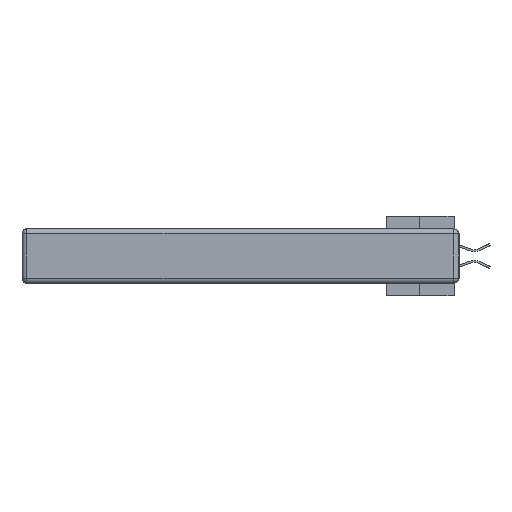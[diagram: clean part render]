
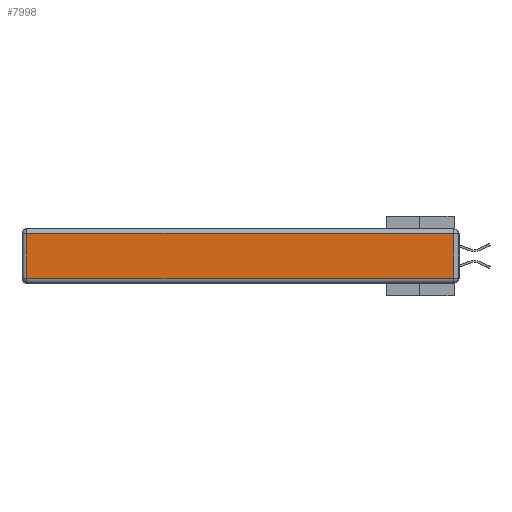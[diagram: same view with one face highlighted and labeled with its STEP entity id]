
A CAD part, left-side view. The second image highlights one B-rep face of the part: STEP entity #7998.
In plain terms, the highlighted planar face has unit normal (-1, 0, 0).
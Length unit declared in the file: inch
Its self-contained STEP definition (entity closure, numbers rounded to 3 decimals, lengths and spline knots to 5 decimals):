
#637 = VERTEX_POINT ( 'NONE', #21173 ) ;
#3758 = LINE ( 'NONE', #36988, #16780 ) ;
#6068 = CARTESIAN_POINT ( 'NONE',  ( 0., 0., -0.313 ) ) ;
#6071 = VECTOR ( 'NONE', #31229, 39.37008 ) ;
#6624 = VERTEX_POINT ( 'NONE', #7556 ) ;
#7320 = LINE ( 'NONE', #24693, #14681 ) ;
#7408 = ORIENTED_EDGE ( 'NONE', *, *, #41758, .T. ) ;
#7542 = CARTESIAN_POINT ( 'NONE',  ( 0., 0., -0.343 ) ) ;
#7556 = CARTESIAN_POINT ( 'NONE',  ( 0., 0.03, -0.03 ) ) ;
#7998 = ADVANCED_FACE ( 'NONE', ( #30467 ), #21424, .T. ) ;
#9216 = LINE ( 'NONE', #45292, #31706 ) ;
#9515 = DIRECTION ( 'NONE',  ( 0., 1., 0. ) ) ;
#10501 = DIRECTION ( 'NONE',  ( -1., 0., 0. ) ) ;
#10829 = DIRECTION ( 'NONE',  ( 0., 0., 1. ) ) ;
#14134 = EDGE_CURVE ( 'NONE', #637, #38287, #3758, .T. ) ;
#14681 = VECTOR ( 'NONE', #41924, 39.37008 ) ;
#16780 = VECTOR ( 'NONE', #43570, 39.37008 ) ;
#19250 = AXIS2_PLACEMENT_3D ( 'NONE', #7542, #10501, #10829 ) ;
#20720 = EDGE_CURVE ( 'NONE', #38287, #21217, #45965, .T. ) ;
#21173 = CARTESIAN_POINT ( 'NONE',  ( 0., 2.72, -0.03 ) ) ;
#21217 = VERTEX_POINT ( 'NONE', #27257 ) ;
#21424 = PLANE ( 'NONE',  #19250 ) ;
#24693 = CARTESIAN_POINT ( 'NONE',  ( 0., 0.03, -0.343 ) ) ;
#25277 = ORIENTED_EDGE ( 'NONE', *, *, #20720, .T. ) ;
#27257 = CARTESIAN_POINT ( 'NONE',  ( 0., 0.03, -0.313 ) ) ;
#28743 = CARTESIAN_POINT ( 'NONE',  ( 0., 2.72, -0.313 ) ) ;
#30467 = FACE_OUTER_BOUND ( 'NONE', #36541, .T. ) ;
#31229 = DIRECTION ( 'NONE',  ( 0., -1., 0. ) ) ;
#31706 = VECTOR ( 'NONE', #9515, 39.37008 ) ;
#36541 = EDGE_LOOP ( 'NONE', ( #25277, #42987, #7408, #43739 ) ) ;
#36988 = CARTESIAN_POINT ( 'NONE',  ( 0., 2.72, -0.343 ) ) ;
#37415 = EDGE_CURVE ( 'NONE', #21217, #6624, #7320, .T. ) ;
#38287 = VERTEX_POINT ( 'NONE', #28743 ) ;
#41758 = EDGE_CURVE ( 'NONE', #6624, #637, #9216, .T. ) ;
#41924 = DIRECTION ( 'NONE',  ( 0., 0., 1. ) ) ;
#42987 = ORIENTED_EDGE ( 'NONE', *, *, #37415, .T. ) ;
#43570 = DIRECTION ( 'NONE',  ( 0., 0., -1. ) ) ;
#43739 = ORIENTED_EDGE ( 'NONE', *, *, #14134, .T. ) ;
#45292 = CARTESIAN_POINT ( 'NONE',  ( 0., 2.75, -0.03 ) ) ;
#45965 = LINE ( 'NONE', #6068, #6071 ) ;
